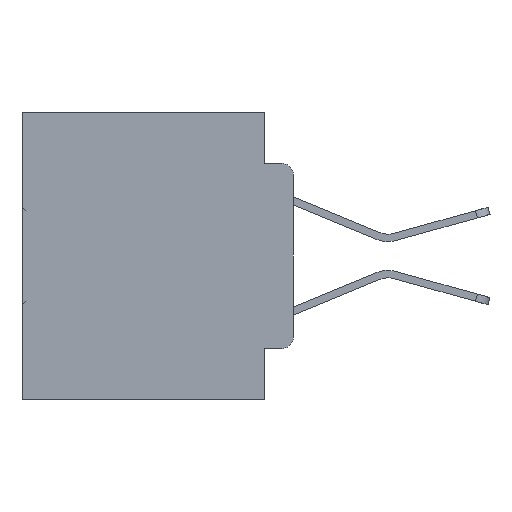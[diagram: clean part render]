
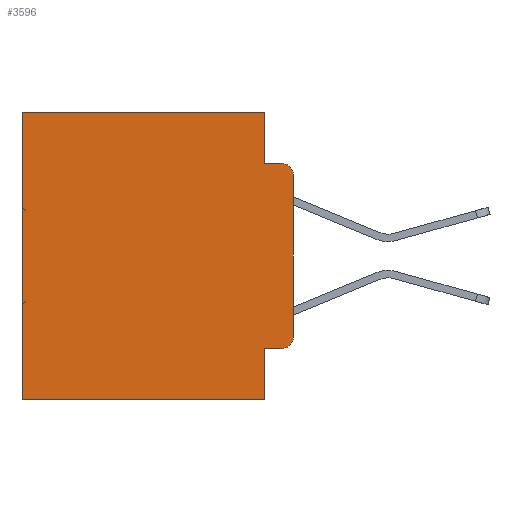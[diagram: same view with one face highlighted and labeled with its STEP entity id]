
A CAD part, left-side view. The second image highlights one B-rep face of the part: STEP entity #3596.
In plain terms, the highlighted planar face has unit normal (-1, 0, 0).
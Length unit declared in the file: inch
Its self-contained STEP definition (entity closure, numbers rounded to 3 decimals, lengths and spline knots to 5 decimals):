
#184 = VERTEX_POINT ( 'NONE', #27141 ) ;
#290 = AXIS2_PLACEMENT_3D ( 'NONE', #23592, #7536, #26228 ) ;
#418 = CARTESIAN_POINT ( 'NONE',  ( 0.298, 0.02, -0.4115 ) ) ;
#593 = DIRECTION ( 'NONE',  ( 1., 0., 0. ) ) ;
#717 = PLANE ( 'NONE',  #26138 ) ;
#926 = CARTESIAN_POINT ( 'NONE',  ( 0.298, 0.473, 0. ) ) ;
#1104 = VERTEX_POINT ( 'NONE', #29912 ) ;
#1652 = CIRCLE ( 'NONE', #22609, 0.02 ) ;
#1968 = VERTEX_POINT ( 'NONE', #5829 ) ;
#1994 = DIRECTION ( 'NONE',  ( 0., -1., 0. ) ) ;
#2144 = CARTESIAN_POINT ( 'NONE',  ( 0.298, 0.051, -0.5 ) ) ;
#2240 = EDGE_CURVE ( 'NONE', #24549, #1968, #25005, .T. ) ;
#2325 = DIRECTION ( 'NONE',  ( 0., 0., -1. ) ) ;
#2470 = CARTESIAN_POINT ( 'NONE',  ( 0.298, 0., -0.1085 ) ) ;
#3335 = ORIENTED_EDGE ( 'NONE', *, *, #8367, .T. ) ;
#3488 = VECTOR ( 'NONE', #14539, 39.37008 ) ;
#3596 = ADVANCED_FACE ( 'NONE', ( #21213 ), #717, .F. ) ;
#5829 = CARTESIAN_POINT ( 'NONE',  ( 0.298, 0., -0.3915 ) ) ;
#5838 = ORIENTED_EDGE ( 'NONE', *, *, #29679, .T. ) ;
#6515 = EDGE_CURVE ( 'NONE', #21941, #32519, #10701, .T. ) ;
#6557 = ORIENTED_EDGE ( 'NONE', *, *, #31751, .F. ) ;
#6813 = VERTEX_POINT ( 'NONE', #23722 ) ;
#7031 = DIRECTION ( 'NONE',  ( 0., 1., 0. ) ) ;
#7536 = DIRECTION ( 'NONE',  ( -1., 0., 0. ) ) ;
#7633 = CARTESIAN_POINT ( 'NONE',  ( 0.298, 0., 0. ) ) ;
#8024 = VECTOR ( 'NONE', #20355, 39.37008 ) ;
#8280 = LINE ( 'NONE', #28927, #21702 ) ;
#8367 = EDGE_CURVE ( 'NONE', #184, #1104, #12734, .T. ) ;
#9855 = VECTOR ( 'NONE', #16364, 39.37008 ) ;
#9933 = CARTESIAN_POINT ( 'NONE',  ( 0.298, 0.051, -0.4115 ) ) ;
#10364 = EDGE_LOOP ( 'NONE', ( #11847, #5838, #16199, #33746, #12808, #3335, #6557, #25747, #16237, #23778 ) ) ;
#10421 = DIRECTION ( 'NONE',  ( 0., 1., 0. ) ) ;
#10701 = LINE ( 'NONE', #14613, #9855 ) ;
#11300 = EDGE_CURVE ( 'NONE', #6813, #184, #8280, .T. ) ;
#11785 = VERTEX_POINT ( 'NONE', #25632 ) ;
#11847 = ORIENTED_EDGE ( 'NONE', *, *, #2240, .F. ) ;
#12390 = CARTESIAN_POINT ( 'NONE',  ( 0.298, 0., -0.5 ) ) ;
#12734 = LINE ( 'NONE', #926, #32809 ) ;
#12808 = ORIENTED_EDGE ( 'NONE', *, *, #11300, .T. ) ;
#14060 = LINE ( 'NONE', #18679, #20325 ) ;
#14459 = CARTESIAN_POINT ( 'NONE',  ( 0.298, 0., 0. ) ) ;
#14539 = DIRECTION ( 'NONE',  ( 0., 0., -1. ) ) ;
#14613 = CARTESIAN_POINT ( 'NONE',  ( 0.298, 0.051, 0. ) ) ;
#15418 = DIRECTION ( 'NONE',  ( 0., 0., -1. ) ) ;
#15527 = CIRCLE ( 'NONE', #290, 0.02 ) ;
#15608 = EDGE_CURVE ( 'NONE', #6813, #11785, #29206, .T. ) ;
#16109 = VECTOR ( 'NONE', #1994, 39.37008 ) ;
#16199 = ORIENTED_EDGE ( 'NONE', *, *, #22723, .F. ) ;
#16237 = ORIENTED_EDGE ( 'NONE', *, *, #33719, .T. ) ;
#16364 = DIRECTION ( 'NONE',  ( 0., 0., -1. ) ) ;
#17690 = CARTESIAN_POINT ( 'NONE',  ( 0.298, 0.051, 0. ) ) ;
#18631 = DIRECTION ( 'NONE',  ( -1., 0., 0. ) ) ;
#18679 = CARTESIAN_POINT ( 'NONE',  ( 0.298, 0.051, -0.0885 ) ) ;
#20325 = VECTOR ( 'NONE', #21344, 39.37008 ) ;
#20355 = DIRECTION ( 'NONE',  ( 0., 0., -1. ) ) ;
#21213 = FACE_OUTER_BOUND ( 'NONE', #10364, .T. ) ;
#21344 = DIRECTION ( 'NONE',  ( 0., -1., 0. ) ) ;
#21702 = VECTOR ( 'NONE', #10421, 39.37008 ) ;
#21941 = VERTEX_POINT ( 'NONE', #9933 ) ;
#22609 = AXIS2_PLACEMENT_3D ( 'NONE', #34133, #18631, #2325 ) ;
#22723 = EDGE_CURVE ( 'NONE', #11785, #30954, #14060, .T. ) ;
#23167 = LINE ( 'NONE', #23497, #16109 ) ;
#23497 = CARTESIAN_POINT ( 'NONE',  ( 0.298, 0.051, -0.4115 ) ) ;
#23592 = CARTESIAN_POINT ( 'NONE',  ( 0.298, 0.02, -0.3915 ) ) ;
#23722 = CARTESIAN_POINT ( 'NONE',  ( 0.298, 0.051, 0. ) ) ;
#23778 = ORIENTED_EDGE ( 'NONE', *, *, #26876, .T. ) ;
#24549 = VERTEX_POINT ( 'NONE', #2470 ) ;
#25005 = LINE ( 'NONE', #14459, #3488 ) ;
#25632 = CARTESIAN_POINT ( 'NONE',  ( 0.298, 0.051, -0.0885 ) ) ;
#25747 = ORIENTED_EDGE ( 'NONE', *, *, #6515, .F. ) ;
#26138 = AXIS2_PLACEMENT_3D ( 'NONE', #7633, #593, #15418 ) ;
#26199 = VECTOR ( 'NONE', #7031, 39.37008 ) ;
#26228 = DIRECTION ( 'NONE',  ( 0., 0., -1. ) ) ;
#26876 = EDGE_CURVE ( 'NONE', #29275, #1968, #15527, .T. ) ;
#27141 = CARTESIAN_POINT ( 'NONE',  ( 0.298, 0.473, 0. ) ) ;
#27610 = CARTESIAN_POINT ( 'NONE',  ( 0.298, 0.02, -0.0885 ) ) ;
#27843 = DIRECTION ( 'NONE',  ( 0., 0., -1. ) ) ;
#28927 = CARTESIAN_POINT ( 'NONE',  ( 0.298, 0., 0. ) ) ;
#29206 = LINE ( 'NONE', #17690, #8024 ) ;
#29275 = VERTEX_POINT ( 'NONE', #418 ) ;
#29679 = EDGE_CURVE ( 'NONE', #24549, #30954, #1652, .T. ) ;
#29912 = CARTESIAN_POINT ( 'NONE',  ( 0.298, 0.473, -0.5 ) ) ;
#30954 = VERTEX_POINT ( 'NONE', #27610 ) ;
#31751 = EDGE_CURVE ( 'NONE', #32519, #1104, #33774, .T. ) ;
#32519 = VERTEX_POINT ( 'NONE', #2144 ) ;
#32809 = VECTOR ( 'NONE', #27843, 39.37008 ) ;
#33719 = EDGE_CURVE ( 'NONE', #21941, #29275, #23167, .T. ) ;
#33746 = ORIENTED_EDGE ( 'NONE', *, *, #15608, .F. ) ;
#33774 = LINE ( 'NONE', #12390, #26199 ) ;
#34133 = CARTESIAN_POINT ( 'NONE',  ( 0.298, 0.02, -0.1085 ) ) ;
